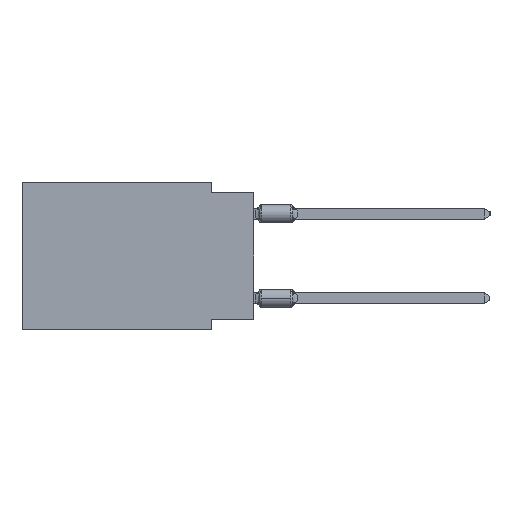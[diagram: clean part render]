
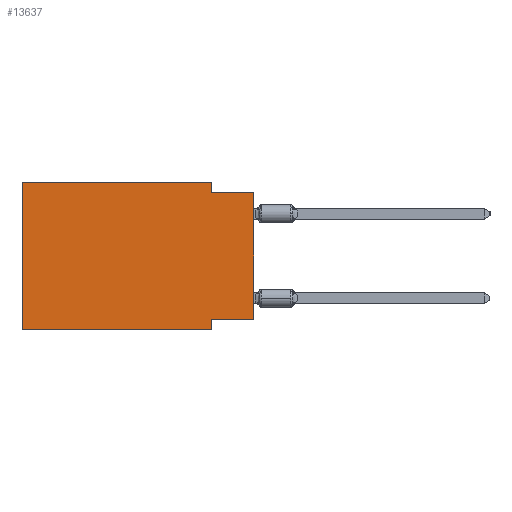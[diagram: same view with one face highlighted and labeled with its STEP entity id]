
A CAD part, left-side view. The second image highlights one B-rep face of the part: STEP entity #13637.
In plain terms, the highlighted planar face has unit normal (-1, 0, 0).
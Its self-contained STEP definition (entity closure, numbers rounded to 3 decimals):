
#1262 = PLANE ( 'NONE',  #43555 ) ;
#1566 = DIRECTION ( 'NONE',  ( 0., 0., -1. ) ) ;
#1887 = CARTESIAN_POINT ( 'NONE',  ( 0., 0., -0.635 ) ) ;
#2063 = LINE ( 'NONE', #48090, #45051 ) ;
#2096 = VERTEX_POINT ( 'NONE', #15158 ) ;
#3023 = DIRECTION ( 'NONE',  ( 0., 0., 1. ) ) ;
#5074 = ORIENTED_EDGE ( 'NONE', *, *, #24315, .F. ) ;
#5787 = EDGE_CURVE ( 'NONE', #11644, #41636, #21024, .T. ) ;
#5929 = ORIENTED_EDGE ( 'NONE', *, *, #51674, .T. ) ;
#6431 = EDGE_LOOP ( 'NONE', ( #52320, #32013, #37273, #27325, #5074, #5929, #38810, #57040 ) ) ;
#9240 = CARTESIAN_POINT ( 'NONE',  ( 0., 2.54, -0.635 ) ) ;
#9395 = CARTESIAN_POINT ( 'NONE',  ( 0., 0., -8.255 ) ) ;
#11644 = VERTEX_POINT ( 'NONE', #51849 ) ;
#12751 = CARTESIAN_POINT ( 'NONE',  ( 0., 0., 0. ) ) ;
#13200 = VECTOR ( 'NONE', #3023, 1000. ) ;
#13230 = DIRECTION ( 'NONE',  ( 0., 1., 0. ) ) ;
#13637 = ADVANCED_FACE ( 'NONE', ( #41683 ), #1262, .F. ) ;
#15158 = CARTESIAN_POINT ( 'NONE',  ( 0., 13.97, -8.89 ) ) ;
#17245 = EDGE_CURVE ( 'NONE', #39710, #41915, #50025, .T. ) ;
#18625 = VECTOR ( 'NONE', #28735, 1000. ) ;
#19282 = CARTESIAN_POINT ( 'NONE',  ( 0., 13.97, 0. ) ) ;
#20085 = VECTOR ( 'NONE', #32617, 1000. ) ;
#21024 = LINE ( 'NONE', #12751, #13200 ) ;
#23461 = CARTESIAN_POINT ( 'NONE',  ( 0., 13.97, 0. ) ) ;
#24315 = EDGE_CURVE ( 'NONE', #2096, #39710, #25289, .T. ) ;
#25289 = LINE ( 'NONE', #57685, #55673 ) ;
#25374 = DIRECTION ( 'NONE',  ( 0., 0., -1. ) ) ;
#25385 = CARTESIAN_POINT ( 'NONE',  ( 0., 2.54, 0. ) ) ;
#26879 = VECTOR ( 'NONE', #13230, 1000. ) ;
#27325 = ORIENTED_EDGE ( 'NONE', *, *, #17245, .F. ) ;
#27761 = CARTESIAN_POINT ( 'NONE',  ( 0., 0., -0.635 ) ) ;
#28452 = CARTESIAN_POINT ( 'NONE',  ( 0., 2.54, -8.89 ) ) ;
#28735 = DIRECTION ( 'NONE',  ( 0., -1., 0. ) ) ;
#31708 = VECTOR ( 'NONE', #58001, 1000. ) ;
#32013 = ORIENTED_EDGE ( 'NONE', *, *, #39145, .F. ) ;
#32229 = EDGE_CURVE ( 'NONE', #52468, #36289, #2063, .T. ) ;
#32617 = DIRECTION ( 'NONE',  ( 0., 0., -1. ) ) ;
#33030 = CARTESIAN_POINT ( 'NONE',  ( 0., 2.54, -8.255 ) ) ;
#34378 = VERTEX_POINT ( 'NONE', #9240 ) ;
#36289 = VERTEX_POINT ( 'NONE', #28452 ) ;
#37273 = ORIENTED_EDGE ( 'NONE', *, *, #51814, .F. ) ;
#38810 = ORIENTED_EDGE ( 'NONE', *, *, #32229, .F. ) ;
#39145 = EDGE_CURVE ( 'NONE', #34378, #41636, #42314, .T. ) ;
#39710 = VERTEX_POINT ( 'NONE', #57076 ) ;
#40029 = LINE ( 'NONE', #44154, #31708 ) ;
#40084 = LINE ( 'NONE', #9395, #26879 ) ;
#41014 = VECTOR ( 'NONE', #45600, 1000. ) ;
#41636 = VERTEX_POINT ( 'NONE', #27761 ) ;
#41683 = FACE_OUTER_BOUND ( 'NONE', #6431, .T. ) ;
#41915 = VERTEX_POINT ( 'NONE', #25385 ) ;
#42314 = LINE ( 'NONE', #1887, #18625 ) ;
#42999 = DIRECTION ( 'NONE',  ( 0., 0., 1. ) ) ;
#43555 = AXIS2_PLACEMENT_3D ( 'NONE', #19282, #55830, #1566 ) ;
#44154 = CARTESIAN_POINT ( 'NONE',  ( 0., 13.97, -8.89 ) ) ;
#45051 = VECTOR ( 'NONE', #25374, 1000. ) ;
#45600 = DIRECTION ( 'NONE',  ( 0., -1., 0. ) ) ;
#45913 = CARTESIAN_POINT ( 'NONE',  ( 0., 2.54, 0. ) ) ;
#48090 = CARTESIAN_POINT ( 'NONE',  ( 0., 2.54, -8.89 ) ) ;
#49997 = EDGE_CURVE ( 'NONE', #11644, #52468, #40084, .T. ) ;
#50025 = LINE ( 'NONE', #23461, #41014 ) ;
#51674 = EDGE_CURVE ( 'NONE', #2096, #36289, #40029, .T. ) ;
#51814 = EDGE_CURVE ( 'NONE', #41915, #34378, #55618, .T. ) ;
#51849 = CARTESIAN_POINT ( 'NONE',  ( 0., 0., -8.255 ) ) ;
#52320 = ORIENTED_EDGE ( 'NONE', *, *, #5787, .T. ) ;
#52468 = VERTEX_POINT ( 'NONE', #33030 ) ;
#55618 = LINE ( 'NONE', #45913, #20085 ) ;
#55673 = VECTOR ( 'NONE', #42999, 1000. ) ;
#55830 = DIRECTION ( 'NONE',  ( 1., 0., 0. ) ) ;
#57040 = ORIENTED_EDGE ( 'NONE', *, *, #49997, .F. ) ;
#57076 = CARTESIAN_POINT ( 'NONE',  ( 0., 13.97, 0. ) ) ;
#57685 = CARTESIAN_POINT ( 'NONE',  ( 0., 13.97, 0. ) ) ;
#58001 = DIRECTION ( 'NONE',  ( 0., -1., 0. ) ) ;
